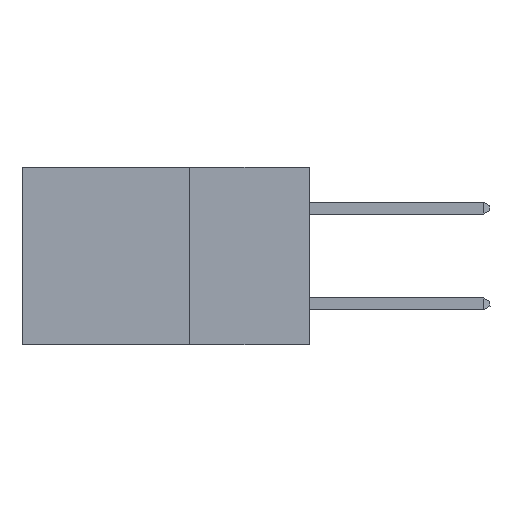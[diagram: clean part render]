
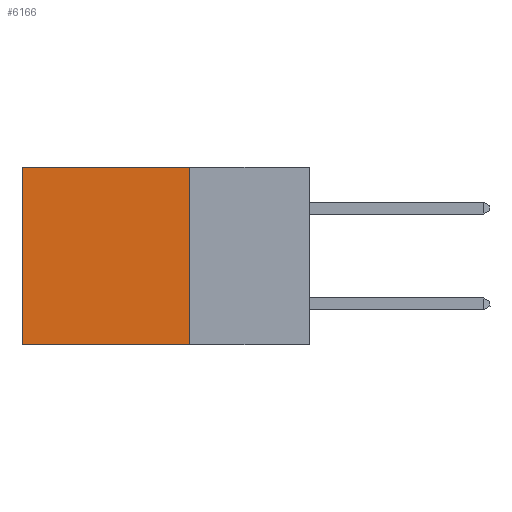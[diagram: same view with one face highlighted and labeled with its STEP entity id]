
A CAD part, left-side view. The second image highlights one B-rep face of the part: STEP entity #6166.
In plain terms, the highlighted planar face has unit normal (-1, 0, 0).
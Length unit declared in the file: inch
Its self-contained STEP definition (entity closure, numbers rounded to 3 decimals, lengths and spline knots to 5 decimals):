
#432 = VERTEX_POINT ( 'NONE', #21126 ) ;
#1482 = AXIS2_PLACEMENT_3D ( 'NONE', #1985, #15491, #5544 ) ;
#1985 = CARTESIAN_POINT ( 'NONE',  ( 0.2875, 0.25, 0. ) ) ;
#2159 = DIRECTION ( 'NONE',  ( 0., 0., -1. ) ) ;
#2411 = ORIENTED_EDGE ( 'NONE', *, *, #12197, .T. ) ;
#2767 = EDGE_CURVE ( 'NONE', #14970, #432, #18268, .T. ) ;
#3786 = VERTEX_POINT ( 'NONE', #21592 ) ;
#3957 = CARTESIAN_POINT ( 'NONE',  ( 0.2875, 0.25, 0. ) ) ;
#4201 = ORIENTED_EDGE ( 'NONE', *, *, #14542, .F. ) ;
#4322 = VERTEX_POINT ( 'NONE', #14778 ) ;
#5216 = DIRECTION ( 'NONE',  ( 0., 1., 0. ) ) ;
#5325 = DIRECTION ( 'NONE',  ( 0., 1., 0. ) ) ;
#5544 = DIRECTION ( 'NONE',  ( 0., 0., -1. ) ) ;
#5622 = DIRECTION ( 'NONE',  ( 0., 0., -1. ) ) ;
#6166 = ADVANCED_FACE ( 'NONE', ( #7656 ), #8793, .F. ) ;
#6490 = LINE ( 'NONE', #20333, #18194 ) ;
#7265 = LINE ( 'NONE', #13505, #15005 ) ;
#7656 = FACE_OUTER_BOUND ( 'NONE', #11348, .T. ) ;
#8301 = ORIENTED_EDGE ( 'NONE', *, *, #2767, .F. ) ;
#8793 = PLANE ( 'NONE',  #1482 ) ;
#9727 = CARTESIAN_POINT ( 'NONE',  ( 0.2875, 0.25, 0. ) ) ;
#11348 = EDGE_LOOP ( 'NONE', ( #2411, #4201, #8301, #20187 ) ) ;
#12197 = EDGE_CURVE ( 'NONE', #4322, #3786, #20909, .T. ) ;
#13087 = VECTOR ( 'NONE', #5622, 39.37008 ) ;
#13505 = CARTESIAN_POINT ( 'NONE',  ( 0.2875, 0.25, -0.37 ) ) ;
#13829 = VECTOR ( 'NONE', #2159, 39.37008 ) ;
#13972 = EDGE_CURVE ( 'NONE', #14970, #4322, #6490, .T. ) ;
#14542 = EDGE_CURVE ( 'NONE', #432, #3786, #7265, .T. ) ;
#14778 = CARTESIAN_POINT ( 'NONE',  ( 0.2875, 0.6, 0. ) ) ;
#14970 = VERTEX_POINT ( 'NONE', #9727 ) ;
#15005 = VECTOR ( 'NONE', #5216, 39.37008 ) ;
#15491 = DIRECTION ( 'NONE',  ( 1., 0., 0. ) ) ;
#17238 = CARTESIAN_POINT ( 'NONE',  ( 0.2875, 0.6, 0. ) ) ;
#18194 = VECTOR ( 'NONE', #5325, 39.37008 ) ;
#18268 = LINE ( 'NONE', #3957, #13829 ) ;
#20187 = ORIENTED_EDGE ( 'NONE', *, *, #13972, .T. ) ;
#20333 = CARTESIAN_POINT ( 'NONE',  ( 0.2875, 0.25, 0. ) ) ;
#20909 = LINE ( 'NONE', #17238, #13087 ) ;
#21126 = CARTESIAN_POINT ( 'NONE',  ( 0.2875, 0.25, -0.37 ) ) ;
#21592 = CARTESIAN_POINT ( 'NONE',  ( 0.2875, 0.6, -0.37 ) ) ;
